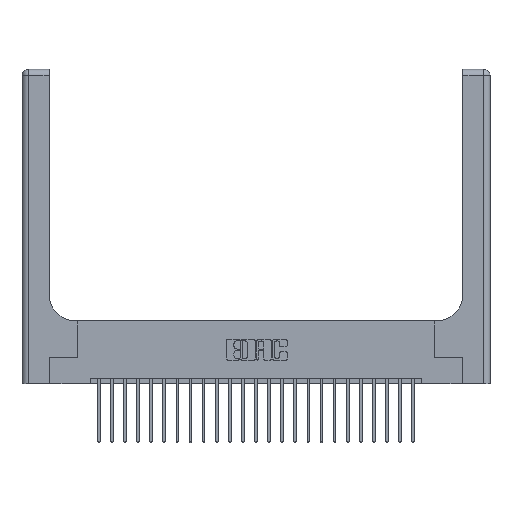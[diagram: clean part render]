
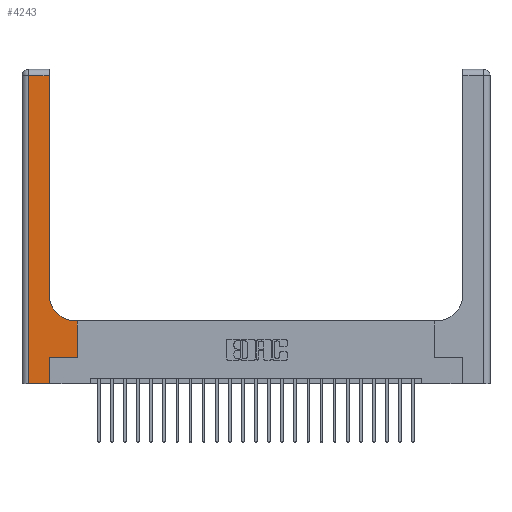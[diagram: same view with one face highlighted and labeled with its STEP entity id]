
A CAD part, top view. The second image highlights one B-rep face of the part: STEP entity #4243.
In plain terms, the highlighted planar face has unit normal (0, 0, 1).
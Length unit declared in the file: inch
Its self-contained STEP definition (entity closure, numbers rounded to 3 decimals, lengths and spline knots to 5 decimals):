
#189 = ORIENTED_EDGE ( 'NONE', *, *, #19845, .T. ) ;
#772 = CARTESIAN_POINT ( 'NONE',  ( 0.528, 0.25, 0.37 ) ) ;
#1213 = CARTESIAN_POINT ( 'NONE',  ( 0.06, 3., 0.37 ) ) ;
#1309 = VECTOR ( 'NONE', #8954, 39.37008 ) ;
#1357 = EDGE_CURVE ( 'NONE', #9036, #3315, #10447, .T. ) ;
#1680 = ORIENTED_EDGE ( 'NONE', *, *, #3940, .T. ) ;
#1754 = ORIENTED_EDGE ( 'NONE', *, *, #1357, .T. ) ;
#1939 = LINE ( 'NONE', #8940, #13935 ) ;
#2125 = CIRCLE ( 'NONE', #2915, 0.25 ) ;
#2915 = AXIS2_PLACEMENT_3D ( 'NONE', #2988, #10469, #16117 ) ;
#2988 = CARTESIAN_POINT ( 'NONE',  ( 0.51, 0.85, 0.37 ) ) ;
#3081 = DIRECTION ( 'NONE',  ( -1., 0., 0. ) ) ;
#3315 = VERTEX_POINT ( 'NONE', #19011 ) ;
#3410 = VERTEX_POINT ( 'NONE', #10155 ) ;
#3940 = EDGE_CURVE ( 'NONE', #7175, #8728, #10067, .T. ) ;
#4060 = VECTOR ( 'NONE', #4643, 39.37008 ) ;
#4243 = ADVANCED_FACE ( 'NONE', ( #20233 ), #16431, .F. ) ;
#4428 = CARTESIAN_POINT ( 'NONE',  ( 0., 2.94, 0.37 ) ) ;
#4504 = EDGE_CURVE ( 'NONE', #9473, #3410, #8677, .T. ) ;
#4536 = CARTESIAN_POINT ( 'NONE',  ( 0.26, 2.94, 0.37 ) ) ;
#4643 = DIRECTION ( 'NONE',  ( 1., 0., 0. ) ) ;
#4811 = CARTESIAN_POINT ( 'NONE',  ( 0.26, 0.6, 0.37 ) ) ;
#6478 = VECTOR ( 'NONE', #10882, 39.37008 ) ;
#6521 = LINE ( 'NONE', #22970, #23001 ) ;
#6848 = CARTESIAN_POINT ( 'NONE',  ( 0.265, 0., 0.37 ) ) ;
#6964 = ORIENTED_EDGE ( 'NONE', *, *, #8185, .T. ) ;
#7175 = VERTEX_POINT ( 'NONE', #4536 ) ;
#7226 = DIRECTION ( 'NONE',  ( 0., 0., -1. ) ) ;
#7993 = DIRECTION ( 'NONE',  ( -1., 0., 0. ) ) ;
#8185 = EDGE_CURVE ( 'NONE', #3315, #13285, #2125, .T. ) ;
#8677 = LINE ( 'NONE', #12476, #13023 ) ;
#8728 = VERTEX_POINT ( 'NONE', #12230 ) ;
#8940 = CARTESIAN_POINT ( 'NONE',  ( 0.528, 0.25, 0.37 ) ) ;
#8954 = DIRECTION ( 'NONE',  ( 0., -1., 0. ) ) ;
#9036 = VERTEX_POINT ( 'NONE', #11109 ) ;
#9073 = CARTESIAN_POINT ( 'NONE',  ( 0., 3., 0.37 ) ) ;
#9473 = VERTEX_POINT ( 'NONE', #21030 ) ;
#9665 = EDGE_LOOP ( 'NONE', ( #189, #1680, #11437, #21700, #13022, #17807, #21228, #1754, #6964 ) ) ;
#9882 = VECTOR ( 'NONE', #7993, 39.37008 ) ;
#10044 = LINE ( 'NONE', #17527, #4060 ) ;
#10067 = LINE ( 'NONE', #4428, #9882 ) ;
#10155 = CARTESIAN_POINT ( 'NONE',  ( 0.265, 0., 0.37 ) ) ;
#10447 = LINE ( 'NONE', #4811, #23875 ) ;
#10469 = DIRECTION ( 'NONE',  ( 0., 0., -1. ) ) ;
#10882 = DIRECTION ( 'NONE',  ( 0., 1., 0. ) ) ;
#10991 = VERTEX_POINT ( 'NONE', #772 ) ;
#11109 = CARTESIAN_POINT ( 'NONE',  ( 0.528, 0.6, 0.37 ) ) ;
#11437 = ORIENTED_EDGE ( 'NONE', *, *, #11595, .T. ) ;
#11595 = EDGE_CURVE ( 'NONE', #8728, #9473, #12866, .T. ) ;
#11806 = EDGE_CURVE ( 'NONE', #18345, #10991, #10044, .T. ) ;
#12230 = CARTESIAN_POINT ( 'NONE',  ( 0.06, 2.94, 0.37 ) ) ;
#12476 = CARTESIAN_POINT ( 'NONE',  ( 0., 0., 0.37 ) ) ;
#12724 = LINE ( 'NONE', #6848, #6478 ) ;
#12866 = LINE ( 'NONE', #1213, #1309 ) ;
#13022 = ORIENTED_EDGE ( 'NONE', *, *, #13248, .T. ) ;
#13023 = VECTOR ( 'NONE', #19614, 39.37008 ) ;
#13248 = EDGE_CURVE ( 'NONE', #3410, #18345, #12724, .T. ) ;
#13285 = VERTEX_POINT ( 'NONE', #21692 ) ;
#13669 = EDGE_CURVE ( 'NONE', #10991, #9036, #1939, .T. ) ;
#13935 = VECTOR ( 'NONE', #20350, 39.37008 ) ;
#16117 = DIRECTION ( 'NONE',  ( 1., 0., 0. ) ) ;
#16223 = CARTESIAN_POINT ( 'NONE',  ( 0.265, 0.25, 0.37 ) ) ;
#16431 = PLANE ( 'NONE',  #23615 ) ;
#17527 = CARTESIAN_POINT ( 'NONE',  ( 0.265, 0.25, 0.37 ) ) ;
#17807 = ORIENTED_EDGE ( 'NONE', *, *, #11806, .T. ) ;
#18345 = VERTEX_POINT ( 'NONE', #16223 ) ;
#18400 = DIRECTION ( 'NONE',  ( -1., 0., 0. ) ) ;
#19011 = CARTESIAN_POINT ( 'NONE',  ( 0.51, 0.6, 0.37 ) ) ;
#19168 = DIRECTION ( 'NONE',  ( 0., 1., 0. ) ) ;
#19614 = DIRECTION ( 'NONE',  ( 1., 0., 0. ) ) ;
#19845 = EDGE_CURVE ( 'NONE', #13285, #7175, #6521, .T. ) ;
#20233 = FACE_OUTER_BOUND ( 'NONE', #9665, .T. ) ;
#20350 = DIRECTION ( 'NONE',  ( 0., 1., 0. ) ) ;
#21030 = CARTESIAN_POINT ( 'NONE',  ( 0.06, 0., 0.37 ) ) ;
#21228 = ORIENTED_EDGE ( 'NONE', *, *, #13669, .T. ) ;
#21692 = CARTESIAN_POINT ( 'NONE',  ( 0.26, 0.85, 0.37 ) ) ;
#21700 = ORIENTED_EDGE ( 'NONE', *, *, #4504, .T. ) ;
#22970 = CARTESIAN_POINT ( 'NONE',  ( 0.26, 3., 0.37 ) ) ;
#23001 = VECTOR ( 'NONE', #19168, 39.37008 ) ;
#23615 = AXIS2_PLACEMENT_3D ( 'NONE', #9073, #7226, #18400 ) ;
#23875 = VECTOR ( 'NONE', #3081, 39.37008 ) ;
